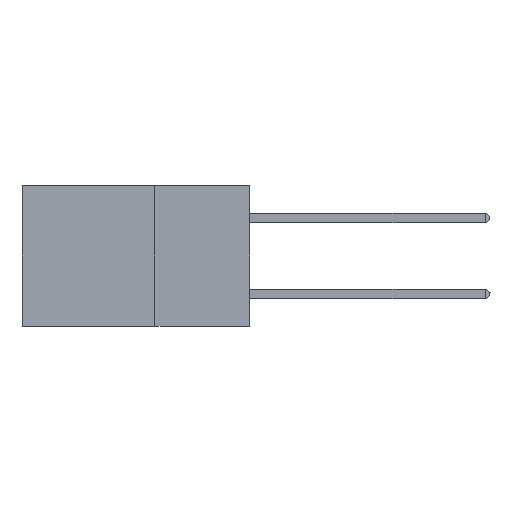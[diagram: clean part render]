
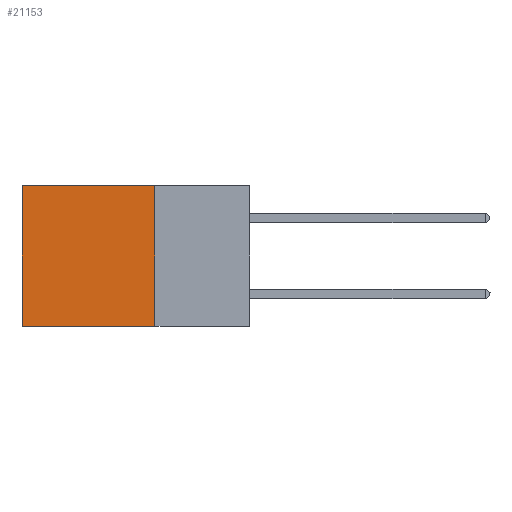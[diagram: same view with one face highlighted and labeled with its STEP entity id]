
A CAD part, left-side view. The second image highlights one B-rep face of the part: STEP entity #21153.
In plain terms, the highlighted planar face has unit normal (-1, 0, 0).
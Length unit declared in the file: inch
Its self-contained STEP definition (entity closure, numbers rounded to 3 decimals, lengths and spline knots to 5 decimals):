
#525 = PLANE ( 'NONE',  #2306 ) ;
#1203 = ORIENTED_EDGE ( 'NONE', *, *, #16505, .T. ) ;
#1787 = FACE_OUTER_BOUND ( 'NONE', #8546, .T. ) ;
#1882 = VECTOR ( 'NONE', #5172, 39.37008 ) ;
#2252 = CARTESIAN_POINT ( 'NONE',  ( 0.2875, 0.6, -0.37 ) ) ;
#2306 = AXIS2_PLACEMENT_3D ( 'NONE', #19457, #6932, #21540 ) ;
#2544 = VECTOR ( 'NONE', #3729, 39.37008 ) ;
#2959 = CARTESIAN_POINT ( 'NONE',  ( 0.2875, 0.25, 0. ) ) ;
#2977 = EDGE_CURVE ( 'NONE', #4990, #13885, #15363, .T. ) ;
#3729 = DIRECTION ( 'NONE',  ( 0., 0., -1. ) ) ;
#4543 = LINE ( 'NONE', #17381, #5208 ) ;
#4674 = CARTESIAN_POINT ( 'NONE',  ( 0.2875, 0.6, 0. ) ) ;
#4804 = DIRECTION ( 'NONE',  ( 0., 0., -1. ) ) ;
#4990 = VERTEX_POINT ( 'NONE', #14501 ) ;
#5172 = DIRECTION ( 'NONE',  ( 0., 1., 0. ) ) ;
#5208 = VECTOR ( 'NONE', #4804, 39.37008 ) ;
#6932 = DIRECTION ( 'NONE',  ( 1., 0., 0. ) ) ;
#7481 = LINE ( 'NONE', #14202, #2544 ) ;
#8546 = EDGE_LOOP ( 'NONE', ( #1203, #25347, #19799, #22975 ) ) ;
#8873 = DIRECTION ( 'NONE',  ( 0., 1., 0. ) ) ;
#13323 = VERTEX_POINT ( 'NONE', #4674 ) ;
#13885 = VERTEX_POINT ( 'NONE', #2252 ) ;
#14202 = CARTESIAN_POINT ( 'NONE',  ( 0.2875, 0.25, 0. ) ) ;
#14501 = CARTESIAN_POINT ( 'NONE',  ( 0.2875, 0.25, -0.37 ) ) ;
#15363 = LINE ( 'NONE', #23472, #25711 ) ;
#16505 = EDGE_CURVE ( 'NONE', #13323, #13885, #4543, .T. ) ;
#16633 = EDGE_CURVE ( 'NONE', #24144, #13323, #18640, .T. ) ;
#17087 = EDGE_CURVE ( 'NONE', #24144, #4990, #7481, .T. ) ;
#17381 = CARTESIAN_POINT ( 'NONE',  ( 0.2875, 0.6, 0. ) ) ;
#17731 = CARTESIAN_POINT ( 'NONE',  ( 0.2875, 0.25, 0. ) ) ;
#18640 = LINE ( 'NONE', #17731, #1882 ) ;
#19457 = CARTESIAN_POINT ( 'NONE',  ( 0.2875, 0.25, 0. ) ) ;
#19799 = ORIENTED_EDGE ( 'NONE', *, *, #17087, .F. ) ;
#21153 = ADVANCED_FACE ( 'NONE', ( #1787 ), #525, .F. ) ;
#21540 = DIRECTION ( 'NONE',  ( 0., 0., -1. ) ) ;
#22975 = ORIENTED_EDGE ( 'NONE', *, *, #16633, .T. ) ;
#23472 = CARTESIAN_POINT ( 'NONE',  ( 0.2875, 0.25, -0.37 ) ) ;
#24144 = VERTEX_POINT ( 'NONE', #2959 ) ;
#25347 = ORIENTED_EDGE ( 'NONE', *, *, #2977, .F. ) ;
#25711 = VECTOR ( 'NONE', #8873, 39.37008 ) ;
